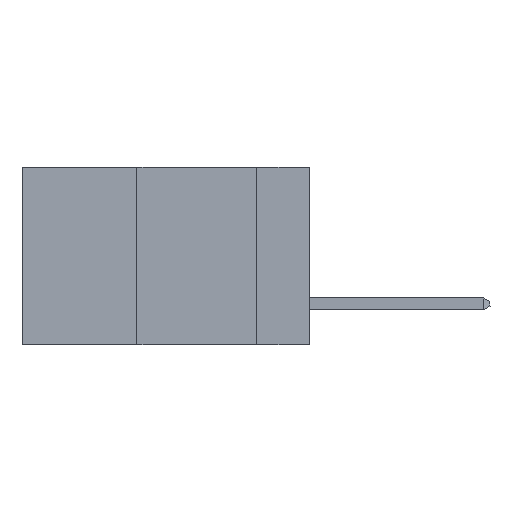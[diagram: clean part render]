
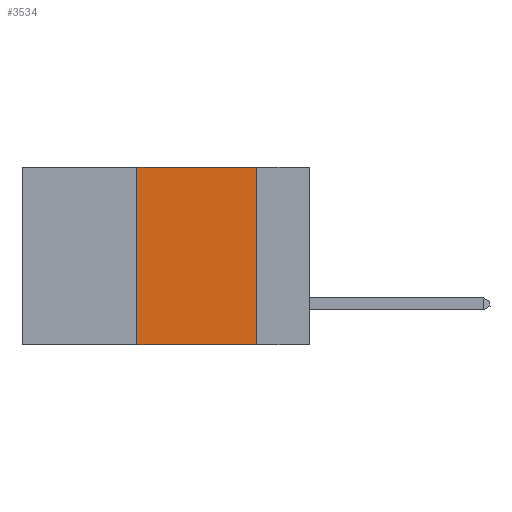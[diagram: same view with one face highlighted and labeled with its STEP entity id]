
A CAD part, left-side view. The second image highlights one B-rep face of the part: STEP entity #3534.
In plain terms, the highlighted planar face has unit normal (-1, 0, 0).
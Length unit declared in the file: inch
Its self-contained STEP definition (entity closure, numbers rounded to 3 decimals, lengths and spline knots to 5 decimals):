
#466 = DIRECTION ( 'NONE',  ( 0., -1., 0. ) ) ;
#728 = DIRECTION ( 'NONE',  ( 0., 0., 1. ) ) ;
#1721 = CARTESIAN_POINT ( 'NONE',  ( 0., 0.6, 0. ) ) ;
#1832 = LINE ( 'NONE', #10804, #11515 ) ;
#1950 = CARTESIAN_POINT ( 'NONE',  ( 0., 0.6, -0.37 ) ) ;
#1996 = CARTESIAN_POINT ( 'NONE',  ( 0., 0.6, 0. ) ) ;
#2476 = VERTEX_POINT ( 'NONE', #6961 ) ;
#2541 = EDGE_CURVE ( 'NONE', #3920, #7763, #8248, .T. ) ;
#3534 = ADVANCED_FACE ( 'NONE', ( #5561 ), #9368, .F. ) ;
#3920 = VERTEX_POINT ( 'NONE', #5812 ) ;
#4352 = EDGE_CURVE ( 'NONE', #6563, #2476, #1832, .T. ) ;
#5561 = FACE_OUTER_BOUND ( 'NONE', #6962, .T. ) ;
#5812 = CARTESIAN_POINT ( 'NONE',  ( 0., 0.36, -0.37 ) ) ;
#6389 = ORIENTED_EDGE ( 'NONE', *, *, #4352, .F. ) ;
#6563 = VERTEX_POINT ( 'NONE', #10930 ) ;
#6961 = CARTESIAN_POINT ( 'NONE',  ( 0., 0.11, -0.37 ) ) ;
#6962 = EDGE_LOOP ( 'NONE', ( #6389, #12472, #9441, #9457 ) ) ;
#7763 = VERTEX_POINT ( 'NONE', #12685 ) ;
#8248 = LINE ( 'NONE', #10357, #8394 ) ;
#8394 = VECTOR ( 'NONE', #728, 39.37008 ) ;
#9107 = LINE ( 'NONE', #1721, #12114 ) ;
#9133 = AXIS2_PLACEMENT_3D ( 'NONE', #1996, #11608, #10362 ) ;
#9368 = PLANE ( 'NONE',  #9133 ) ;
#9409 = EDGE_CURVE ( 'NONE', #7763, #6563, #9107, .T. ) ;
#9441 = ORIENTED_EDGE ( 'NONE', *, *, #2541, .F. ) ;
#9457 = ORIENTED_EDGE ( 'NONE', *, *, #13326, .T. ) ;
#10357 = CARTESIAN_POINT ( 'NONE',  ( 0., 0.36, 0. ) ) ;
#10362 = DIRECTION ( 'NONE',  ( 0., 0., -1. ) ) ;
#10804 = CARTESIAN_POINT ( 'NONE',  ( 0., 0.11, 0. ) ) ;
#10930 = CARTESIAN_POINT ( 'NONE',  ( 0., 0.11, 0. ) ) ;
#11515 = VECTOR ( 'NONE', #12846, 39.37008 ) ;
#11521 = DIRECTION ( 'NONE',  ( 0., -1., 0. ) ) ;
#11608 = DIRECTION ( 'NONE',  ( 1., 0., 0. ) ) ;
#12114 = VECTOR ( 'NONE', #466, 39.37008 ) ;
#12213 = VECTOR ( 'NONE', #11521, 39.37008 ) ;
#12472 = ORIENTED_EDGE ( 'NONE', *, *, #9409, .F. ) ;
#12685 = CARTESIAN_POINT ( 'NONE',  ( 0., 0.36, 0. ) ) ;
#12846 = DIRECTION ( 'NONE',  ( 0., 0., -1. ) ) ;
#13326 = EDGE_CURVE ( 'NONE', #3920, #2476, #13552, .T. ) ;
#13552 = LINE ( 'NONE', #1950, #12213 ) ;
